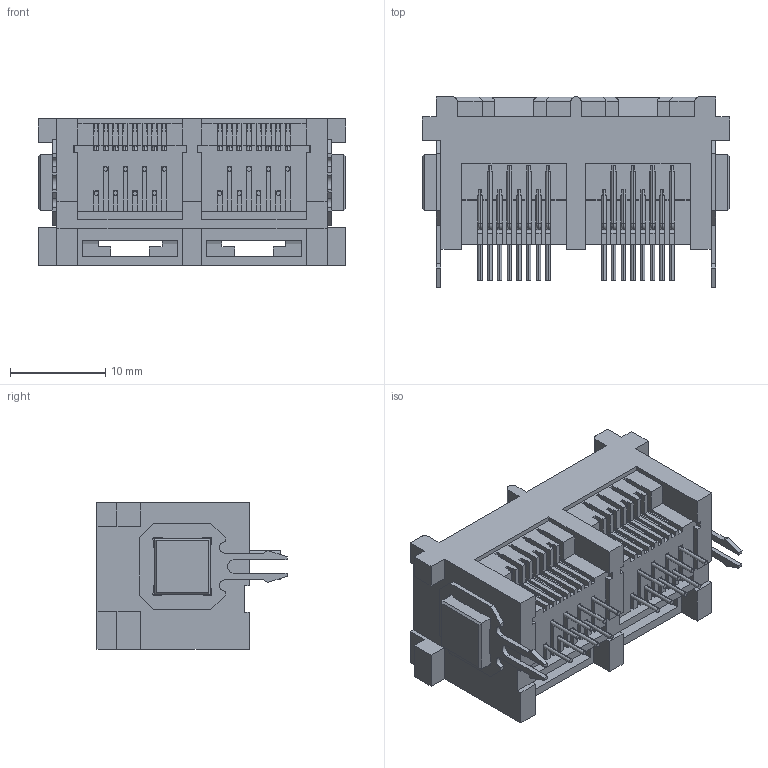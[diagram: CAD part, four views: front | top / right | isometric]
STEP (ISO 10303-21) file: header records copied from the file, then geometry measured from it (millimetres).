
FILE_DESCRIPTION (( 'STEP AP203' ), '1' );
FILE_NAME ('RJF2028821N00033.STEP', '2020-01-20T18:22:32', ( '' ), ( '' ), 'SwSTEP 2.0', 'SolidWorks 2016', '' );
FILE_SCHEMA (( 'CONFIG_CONTROL_DESIGN' ));
Length unit declared in the file: millimetre
Products named in the file (5): F2 Contacts; RJF2028821N00033; F2 Contact Lock; F2 Boardlocks; F2 Insulator
Assembly tree (6 placements, depth 2):
  RJF2028821N00033
    F2 Insulator
    F2 Contacts  x2
    F2 Contact Lock  x2
    F2 Boardlocks
Bounding box: 32.28 x 19.97 x 15.4 mm (x, y, z)
Volume: 3518.9 mm3; surface area: 6910 mm2
Topology: 21 solids, 21 shells, 1130 faces, 3232 edges, 2044 vertices
Faces by surface type: plane 734, cylinder 300, bspline 96
Entity records: 28132 total; most frequent: CARTESIAN_POINT 6146, ORIENTED_EDGE 4684, DIRECTION 4203, EDGE_CURVE 2342, LINE 1913, VECTOR 1913, VERTEX_POINT 1520, AXIS2_PLACEMENT_3D 1145
